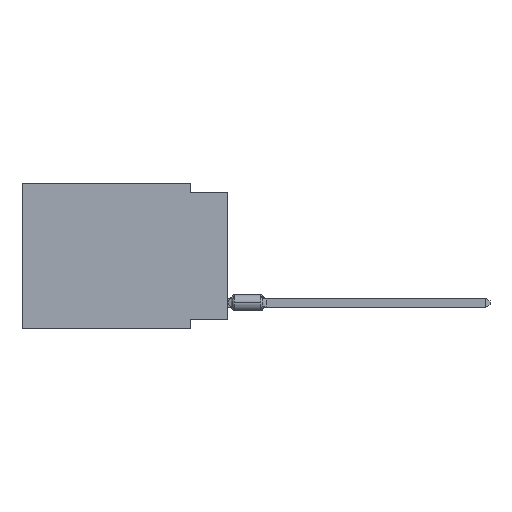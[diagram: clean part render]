
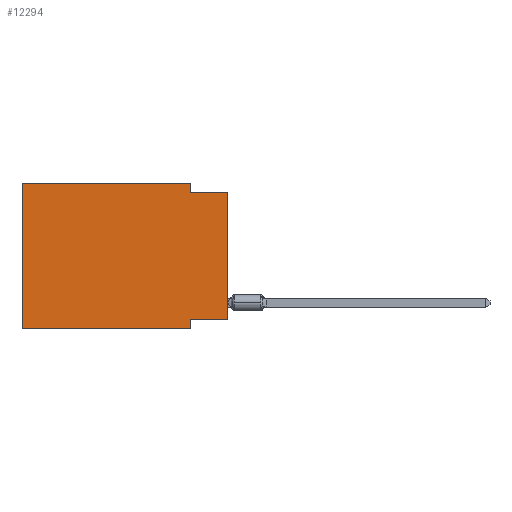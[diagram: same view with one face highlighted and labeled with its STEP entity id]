
A CAD part, left-side view. The second image highlights one B-rep face of the part: STEP entity #12294.
In plain terms, the highlighted planar face has unit normal (-1, 0, 0).
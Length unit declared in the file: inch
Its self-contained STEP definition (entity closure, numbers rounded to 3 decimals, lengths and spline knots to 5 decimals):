
#857 = VECTOR ( 'NONE', #8722, 39.37008 ) ;
#926 = CARTESIAN_POINT ( 'NONE',  ( 0., 0.55, -0.39 ) ) ;
#978 = ORIENTED_EDGE ( 'NONE', *, *, #15716, .F. ) ;
#982 = VERTEX_POINT ( 'NONE', #5726 ) ;
#1433 = EDGE_CURVE ( 'NONE', #982, #6147, #1461, .T. ) ;
#1461 = LINE ( 'NONE', #14405, #17313 ) ;
#1473 = VERTEX_POINT ( 'NONE', #15777 ) ;
#1812 = DIRECTION ( 'NONE',  ( 0., 0., -1. ) ) ;
#1868 = LINE ( 'NONE', #11870, #857 ) ;
#1985 = VECTOR ( 'NONE', #3645, 39.37008 ) ;
#1989 = CARTESIAN_POINT ( 'NONE',  ( 0., 0., -0.365 ) ) ;
#2097 = EDGE_CURVE ( 'NONE', #5592, #3251, #8852, .T. ) ;
#2437 = ORIENTED_EDGE ( 'NONE', *, *, #10555, .F. ) ;
#3100 = AXIS2_PLACEMENT_3D ( 'NONE', #14890, #14984, #14725 ) ;
#3251 = VERTEX_POINT ( 'NONE', #5706 ) ;
#3384 = LINE ( 'NONE', #14678, #4911 ) ;
#3425 = DIRECTION ( 'NONE',  ( 0., -1., 0. ) ) ;
#3613 = FACE_OUTER_BOUND ( 'NONE', #9286, .T. ) ;
#3645 = DIRECTION ( 'NONE',  ( 0., 1., 0. ) ) ;
#3686 = CARTESIAN_POINT ( 'NONE',  ( 0., 0.1, -0.39 ) ) ;
#4806 = LINE ( 'NONE', #5069, #13796 ) ;
#4911 = VECTOR ( 'NONE', #15882, 39.37008 ) ;
#5005 = PLANE ( 'NONE',  #3100 ) ;
#5069 = CARTESIAN_POINT ( 'NONE',  ( 0., 0., -0.025 ) ) ;
#5263 = CARTESIAN_POINT ( 'NONE',  ( 0., 0., 0. ) ) ;
#5592 = VERTEX_POINT ( 'NONE', #8414 ) ;
#5680 = VERTEX_POINT ( 'NONE', #16618 ) ;
#5706 = CARTESIAN_POINT ( 'NONE',  ( 0., 0.1, -0.025 ) ) ;
#5726 = CARTESIAN_POINT ( 'NONE',  ( 0., 0.1, -0.365 ) ) ;
#6098 = CARTESIAN_POINT ( 'NONE',  ( 0., 0.55, 0. ) ) ;
#6147 = VERTEX_POINT ( 'NONE', #3686 ) ;
#6482 = ORIENTED_EDGE ( 'NONE', *, *, #1433, .F. ) ;
#6748 = ORIENTED_EDGE ( 'NONE', *, *, #2097, .F. ) ;
#6880 = EDGE_CURVE ( 'NONE', #5680, #982, #9020, .T. ) ;
#7598 = LINE ( 'NONE', #926, #17403 ) ;
#8414 = CARTESIAN_POINT ( 'NONE',  ( 0., 0.1, 0. ) ) ;
#8507 = VECTOR ( 'NONE', #1812, 39.37008 ) ;
#8665 = DIRECTION ( 'NONE',  ( 0., 0., -1. ) ) ;
#8722 = DIRECTION ( 'NONE',  ( 0., 0., 1. ) ) ;
#8852 = LINE ( 'NONE', #14499, #8507 ) ;
#9020 = LINE ( 'NONE', #1989, #1985 ) ;
#9286 = EDGE_LOOP ( 'NONE', ( #15243, #10371, #6748, #978, #2437, #18085, #6482, #13376 ) ) ;
#10371 = ORIENTED_EDGE ( 'NONE', *, *, #17020, .F. ) ;
#10555 = EDGE_CURVE ( 'NONE', #13552, #15272, #1868, .T. ) ;
#10918 = DIRECTION ( 'NONE',  ( 0., 0., 1. ) ) ;
#11140 = EDGE_CURVE ( 'NONE', #13552, #6147, #7598, .T. ) ;
#11870 = CARTESIAN_POINT ( 'NONE',  ( 0., 0.55, 0. ) ) ;
#12014 = DIRECTION ( 'NONE',  ( 0., -1., 0. ) ) ;
#12294 = ADVANCED_FACE ( 'NONE', ( #3613 ), #5005, .F. ) ;
#13376 = ORIENTED_EDGE ( 'NONE', *, *, #6880, .F. ) ;
#13552 = VERTEX_POINT ( 'NONE', #14810 ) ;
#13786 = EDGE_CURVE ( 'NONE', #5680, #1473, #17930, .T. ) ;
#13796 = VECTOR ( 'NONE', #12014, 39.37008 ) ;
#14405 = CARTESIAN_POINT ( 'NONE',  ( 0., 0.1, -0.39 ) ) ;
#14499 = CARTESIAN_POINT ( 'NONE',  ( 0., 0.1, 0. ) ) ;
#14678 = CARTESIAN_POINT ( 'NONE',  ( 0., 0.55, 0. ) ) ;
#14725 = DIRECTION ( 'NONE',  ( 0., 0., -1. ) ) ;
#14810 = CARTESIAN_POINT ( 'NONE',  ( 0., 0.55, -0.39 ) ) ;
#14890 = CARTESIAN_POINT ( 'NONE',  ( 0., 0.55, 0. ) ) ;
#14984 = DIRECTION ( 'NONE',  ( 1., 0., 0. ) ) ;
#15243 = ORIENTED_EDGE ( 'NONE', *, *, #13786, .T. ) ;
#15272 = VERTEX_POINT ( 'NONE', #6098 ) ;
#15716 = EDGE_CURVE ( 'NONE', #15272, #5592, #3384, .T. ) ;
#15777 = CARTESIAN_POINT ( 'NONE',  ( 0., 0., -0.025 ) ) ;
#15832 = VECTOR ( 'NONE', #10918, 39.37008 ) ;
#15882 = DIRECTION ( 'NONE',  ( 0., -1., 0. ) ) ;
#16618 = CARTESIAN_POINT ( 'NONE',  ( 0., 0., -0.365 ) ) ;
#17020 = EDGE_CURVE ( 'NONE', #3251, #1473, #4806, .T. ) ;
#17313 = VECTOR ( 'NONE', #8665, 39.37008 ) ;
#17403 = VECTOR ( 'NONE', #3425, 39.37008 ) ;
#17930 = LINE ( 'NONE', #5263, #15832 ) ;
#18085 = ORIENTED_EDGE ( 'NONE', *, *, #11140, .T. ) ;
